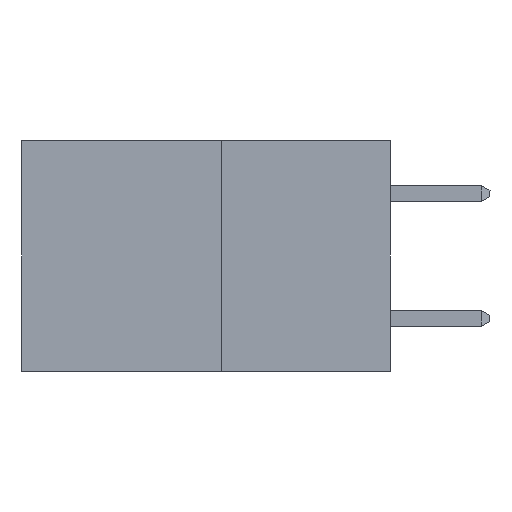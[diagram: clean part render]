
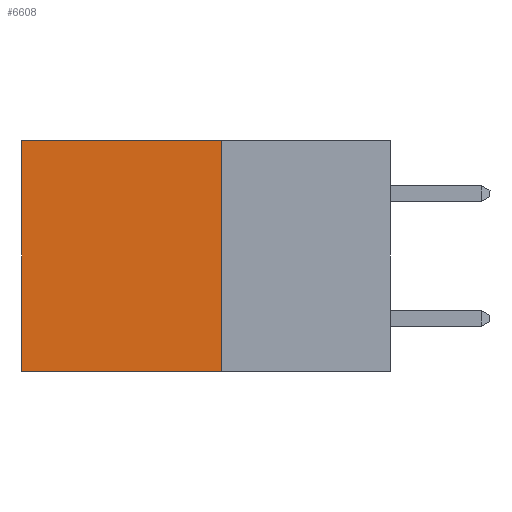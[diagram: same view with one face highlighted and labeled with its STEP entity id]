
A CAD part, left-side view. The second image highlights one B-rep face of the part: STEP entity #6608.
In plain terms, the highlighted planar face has unit normal (-1, 0, 0).
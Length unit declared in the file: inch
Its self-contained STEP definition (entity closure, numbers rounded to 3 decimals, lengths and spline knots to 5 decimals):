
#120 = EDGE_CURVE ( 'NONE', #8152, #1786, #6408, .T. ) ;
#560 = CARTESIAN_POINT ( 'NONE',  ( 0.277, 0.59, -0.37 ) ) ;
#578 = DIRECTION ( 'NONE',  ( 0., 0., -1. ) ) ;
#702 = VERTEX_POINT ( 'NONE', #1317 ) ;
#1070 = EDGE_CURVE ( 'NONE', #1786, #702, #13615, .T. ) ;
#1209 = EDGE_CURVE ( 'NONE', #8152, #1327, #9425, .T. ) ;
#1317 = CARTESIAN_POINT ( 'NONE',  ( 0.277, 0.59, -0.37 ) ) ;
#1327 = VERTEX_POINT ( 'NONE', #13009 ) ;
#1599 = EDGE_CURVE ( 'NONE', #1327, #702, #4787, .T. ) ;
#1786 = VERTEX_POINT ( 'NONE', #12085 ) ;
#1898 = ORIENTED_EDGE ( 'NONE', *, *, #1209, .T. ) ;
#2280 = CARTESIAN_POINT ( 'NONE',  ( 0.277, 0.27, 0. ) ) ;
#3421 = VECTOR ( 'NONE', #13450, 39.37008 ) ;
#3629 = DIRECTION ( 'NONE',  ( 0., 1., 0. ) ) ;
#3721 = EDGE_LOOP ( 'NONE', ( #11797, #13889, #13168, #1898 ) ) ;
#4787 = LINE ( 'NONE', #560, #10455 ) ;
#5740 = CARTESIAN_POINT ( 'NONE',  ( 0.277, 0.27, 0. ) ) ;
#6408 = LINE ( 'NONE', #12640, #3421 ) ;
#6536 = CARTESIAN_POINT ( 'NONE',  ( 0.277, 0.27, -0.37 ) ) ;
#6608 = ADVANCED_FACE ( 'NONE', ( #13800 ), #12119, .F. ) ;
#8152 = VERTEX_POINT ( 'NONE', #2280 ) ;
#9076 = VECTOR ( 'NONE', #13547, 39.37008 ) ;
#9425 = LINE ( 'NONE', #5740, #9076 ) ;
#10455 = VECTOR ( 'NONE', #578, 39.37008 ) ;
#11797 = ORIENTED_EDGE ( 'NONE', *, *, #1599, .T. ) ;
#11975 = DIRECTION ( 'NONE',  ( 0., 0., -1. ) ) ;
#11990 = DIRECTION ( 'NONE',  ( 1., 0., 0. ) ) ;
#12085 = CARTESIAN_POINT ( 'NONE',  ( 0.277, 0.27, -0.37 ) ) ;
#12099 = CARTESIAN_POINT ( 'NONE',  ( 0.277, 0.27, -0.37 ) ) ;
#12119 = PLANE ( 'NONE',  #14564 ) ;
#12640 = CARTESIAN_POINT ( 'NONE',  ( 0.277, 0.27, -0.37 ) ) ;
#12910 = VECTOR ( 'NONE', #3629, 39.37008 ) ;
#13009 = CARTESIAN_POINT ( 'NONE',  ( 0.277, 0.59, 0. ) ) ;
#13168 = ORIENTED_EDGE ( 'NONE', *, *, #120, .F. ) ;
#13450 = DIRECTION ( 'NONE',  ( 0., 0., -1. ) ) ;
#13547 = DIRECTION ( 'NONE',  ( 0., 1., 0. ) ) ;
#13615 = LINE ( 'NONE', #6536, #12910 ) ;
#13800 = FACE_OUTER_BOUND ( 'NONE', #3721, .T. ) ;
#13889 = ORIENTED_EDGE ( 'NONE', *, *, #1070, .F. ) ;
#14564 = AXIS2_PLACEMENT_3D ( 'NONE', #12099, #11990, #11975 ) ;
